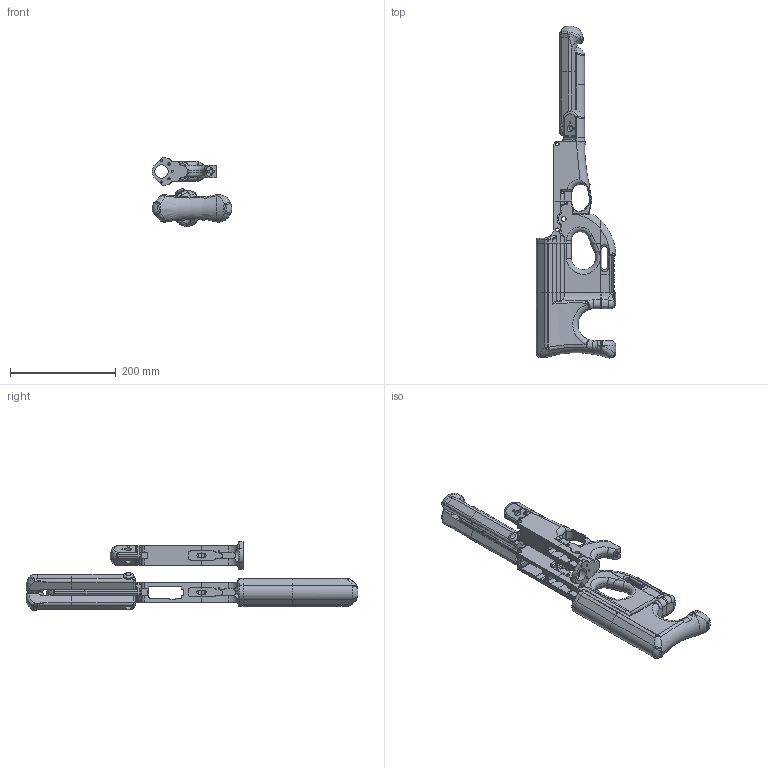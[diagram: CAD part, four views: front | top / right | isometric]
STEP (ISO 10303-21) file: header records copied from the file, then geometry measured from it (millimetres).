
FILE_DESCRIPTION (( 'STEP AP214' ), '1' );
FILE_NAME ('Atlas_Assembly_V2.STEP', '2016-01-25T18:32:09', ( 'WarFairy' ), ( '' ), 'SwSTEP 2.0', 'SolidWorks 2015', '' );
FILE_SCHEMA (( 'AUTOMOTIVE_DESIGN' ));
Length unit declared in the file: inch
Products named in the file (19): Long_Fore_Arm_Part_1_V2; Bipod_Right_Part_2_V2; Bipod_Right_Part_1_V2; Bipod_Peg_Part_2_V2; Bipod_Peg_Part_1_V2; Bipod_Left_Part_2_V2; Bipod_Left_Part_1_V2; Atlas_SSR_Receiver_Rear_V2; Atlas_SSR_Receiver_Front_V2; Atlas_DMR_Receiver_Rear_V2; Atlas_DMR_Receiver_Front_V2; Atlas_Assembly_V2; Stock_Rear_V2; Stock_Rail_Rear_V2; Stock_Rail_Front_V2; Stock_Knob_V2; Stock_Front_V2; Short_Fore_Arm_V2; Long_Fore_Arm_Part_2_V2
Assembly tree (18 placements, depth 2):
  Atlas_Assembly_V2
    Atlas_DMR_Receiver_Front_V2
    Atlas_DMR_Receiver_Rear_V2
    Atlas_SSR_Receiver_Front_V2
    Atlas_SSR_Receiver_Rear_V2
    Bipod_Left_Part_1_V2
    Bipod_Left_Part_2_V2
    Bipod_Peg_Part_1_V2
    Bipod_Peg_Part_2_V2
    Bipod_Right_Part_1_V2
    Bipod_Right_Part_2_V2
    Long_Fore_Arm_Part_1_V2
    Long_Fore_Arm_Part_2_V2
    Short_Fore_Arm_V2
    Stock_Front_V2
    Stock_Knob_V2
    Stock_Rail_Front_V2
    Stock_Rail_Rear_V2
    Stock_Rear_V2
Bounding box: 150.68 x 628.82 x 130.19 mm (x, y, z)
Volume: 1793782.9 mm3; surface area: 311971.1 mm2
Topology: 18 solids, 18 shells, 1646 faces, 4537 edges, 2735 vertices
Faces by surface type: cylinder 496, plane 397, bspline 342, sphere 213, torus 198
Full cylindrical faces by diameter (mm): 3.175 x4, 3.969 x8, 5.182 x1, 6.375 x4, 6.477 x1, 6.858 x4, 7.938 x1, 9.525 x4, 12 x7, 13.5 x1, 18.5 x1, 25.654 x4
Entity records: 80939 total; most frequent: CARTESIAN_POINT 43950, ORIENTED_EDGE 7888, DIRECTION 6936, EDGE_CURVE 3944, AXIS2_PLACEMENT_3D 2762, VERTEX_POINT 2509, EDGE_LOOP 1893, FACE_OUTER_BOUND 1689
